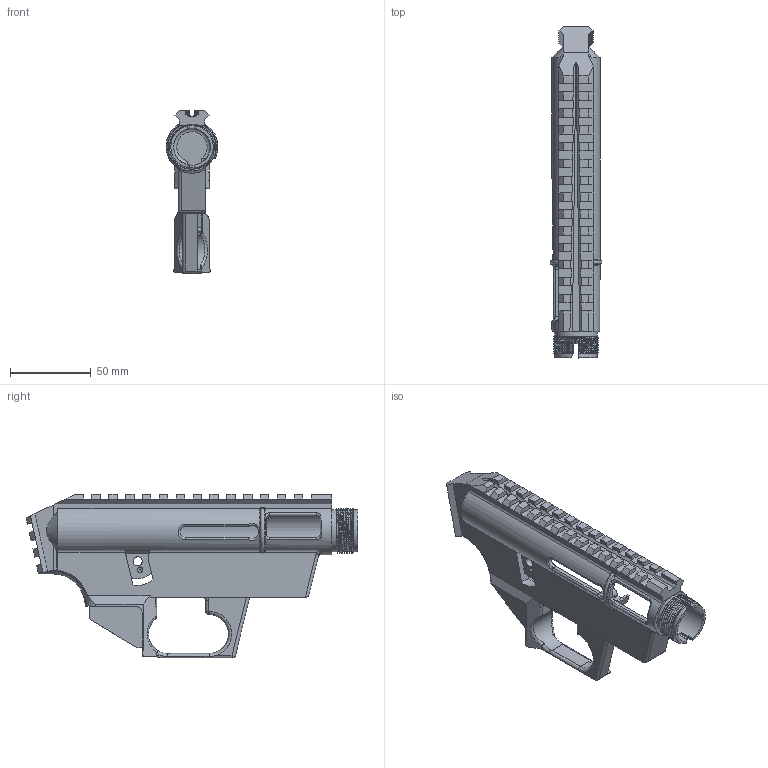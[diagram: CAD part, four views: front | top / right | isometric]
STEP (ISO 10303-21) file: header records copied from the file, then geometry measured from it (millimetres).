
FILE_DESCRIPTION(/* description */ (''),/* implementation_level */ '2;1');
FILE_NAME(/* name */ 'AR-7 Camper III.step',/* time_stamp */ '2021-09-24T21:35:19-04:00',/* author */ (''),/* organization */ (''),/* preprocessor_version */ 'ST-DEVELOPER v18.1',/* originating_system */ 'Autodesk Translation Framework v10.10.0.1391',/* authorisation */ '');
FILE_SCHEMA (('AUTOMOTIVE_DESIGN { 1 0 10303 214 3 1 1 }'));
Length unit declared in the file: millimetre
Products named in the file (1): AR-7 Camper III
Bounding box: 32.28 x 206.17 x 101.34 mm (x, y, z)
Volume: 133479.6 mm3; surface area: 55339.6 mm2
Topology: 3 solids, 3 shells, 591 faces, 1643 edges, 1055 vertices
Faces by surface type: plane 365, cylinder 128, bspline 63, torus 20, cone 11, sphere 4
Full cylindrical faces by diameter (mm): 3.45 x3, 3.65 x1, 4.3 x1, 5.5 x1, 5.65 x1, 7.75 x1, 22.9 x2, 26.132 x2, 26.3 x1, 27.85 x3
Entity records: 22773 total; most frequent: CARTESIAN_POINT 8010, ORIENTED_EDGE 3282, DIRECTION 2785, EDGE_CURVE 1641, LINE 1113, VECTOR 1113, VERTEX_POINT 1055, AXIS2_PLACEMENT_3D 836
